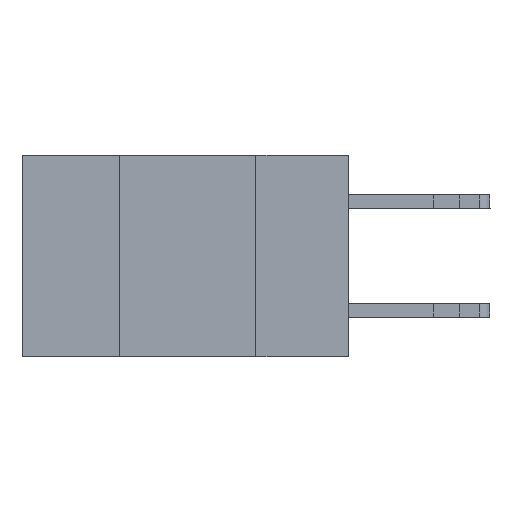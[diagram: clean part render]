
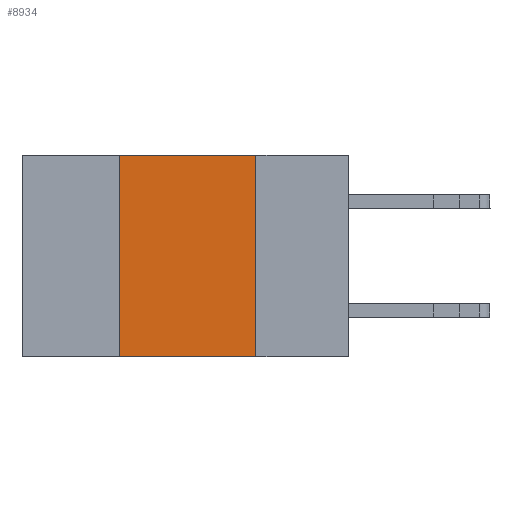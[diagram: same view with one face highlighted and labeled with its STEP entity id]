
A CAD part, left-side view. The second image highlights one B-rep face of the part: STEP entity #8934.
In plain terms, the highlighted planar face has unit normal (-1, 0, 0).
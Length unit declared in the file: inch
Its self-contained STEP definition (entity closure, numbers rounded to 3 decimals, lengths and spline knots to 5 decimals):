
#128 = DIRECTION ( 'NONE',  ( 0., 0., -1. ) ) ;
#209 = DIRECTION ( 'NONE',  ( 0., 0., -1. ) ) ;
#1534 = VERTEX_POINT ( 'NONE', #15031 ) ;
#1869 = DIRECTION ( 'NONE',  ( 0., -1., 0. ) ) ;
#2666 = AXIS2_PLACEMENT_3D ( 'NONE', #15557, #13685, #128 ) ;
#3178 = CARTESIAN_POINT ( 'NONE',  ( 0., 0.17, -0.37 ) ) ;
#4597 = EDGE_CURVE ( 'NONE', #1534, #11159, #14895, .T. ) ;
#4832 = LINE ( 'NONE', #15424, #15842 ) ;
#5961 = ORIENTED_EDGE ( 'NONE', *, *, #17854, .F. ) ;
#6239 = ORIENTED_EDGE ( 'NONE', *, *, #15969, .F. ) ;
#7950 = FACE_OUTER_BOUND ( 'NONE', #17203, .T. ) ;
#8273 = VERTEX_POINT ( 'NONE', #13608 ) ;
#8437 = CARTESIAN_POINT ( 'NONE',  ( 0., 0.17, 0. ) ) ;
#8739 = CARTESIAN_POINT ( 'NONE',  ( 0., 0.6, -0.37 ) ) ;
#8934 = ADVANCED_FACE ( 'NONE', ( #7950 ), #12495, .F. ) ;
#10462 = DIRECTION ( 'NONE',  ( 0., 0., 1. ) ) ;
#10729 = CARTESIAN_POINT ( 'NONE',  ( 0., 0.42, 0. ) ) ;
#10746 = CARTESIAN_POINT ( 'NONE',  ( 0., 0.42, -0.37 ) ) ;
#11159 = VERTEX_POINT ( 'NONE', #10729 ) ;
#11559 = ORIENTED_EDGE ( 'NONE', *, *, #18448, .T. ) ;
#12265 = VECTOR ( 'NONE', #10462, 39.37008 ) ;
#12276 = LINE ( 'NONE', #3178, #16743 ) ;
#12495 = PLANE ( 'NONE',  #2666 ) ;
#13004 = ORIENTED_EDGE ( 'NONE', *, *, #4597, .F. ) ;
#13180 = LINE ( 'NONE', #8739, #13653 ) ;
#13608 = CARTESIAN_POINT ( 'NONE',  ( 0., 0.17, -0.37 ) ) ;
#13653 = VECTOR ( 'NONE', #16140, 39.37008 ) ;
#13685 = DIRECTION ( 'NONE',  ( 1., 0., 0. ) ) ;
#14895 = LINE ( 'NONE', #10746, #12265 ) ;
#15031 = CARTESIAN_POINT ( 'NONE',  ( 0., 0.42, -0.37 ) ) ;
#15424 = CARTESIAN_POINT ( 'NONE',  ( 0., 0.6, 0. ) ) ;
#15557 = CARTESIAN_POINT ( 'NONE',  ( 0., 0.6, 0. ) ) ;
#15842 = VECTOR ( 'NONE', #1869, 39.37008 ) ;
#15969 = EDGE_CURVE ( 'NONE', #17396, #8273, #12276, .T. ) ;
#16140 = DIRECTION ( 'NONE',  ( 0., -1., 0. ) ) ;
#16743 = VECTOR ( 'NONE', #209, 39.37008 ) ;
#17203 = EDGE_LOOP ( 'NONE', ( #6239, #5961, #13004, #11559 ) ) ;
#17396 = VERTEX_POINT ( 'NONE', #8437 ) ;
#17854 = EDGE_CURVE ( 'NONE', #11159, #17396, #4832, .T. ) ;
#18448 = EDGE_CURVE ( 'NONE', #1534, #8273, #13180, .T. ) ;
